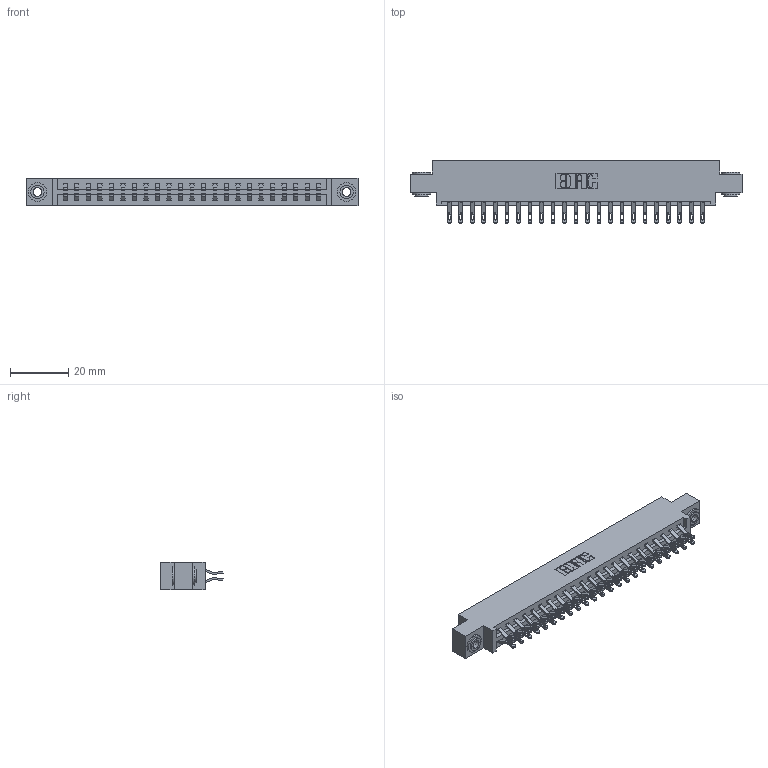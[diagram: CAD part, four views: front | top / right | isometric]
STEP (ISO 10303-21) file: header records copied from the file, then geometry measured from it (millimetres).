
FILE_DESCRIPTION (( 'STEP AP203' ), '1' );
FILE_NAME ('387-046-555-803.STEP', '2019-10-18T08:10:55', ( '' ), ( '' ), 'SwSTEP 2.0', 'SolidWorks 2016', '' );
FILE_SCHEMA (( 'CONFIG_CONTROL_DESIGN' ));
Length unit declared in the file: inch
Products named in the file (4): 337 Part_0.170 Offset - 0.156 Dia-TH; 345-250-002_345-250-002-102; 387-046-555-803; 345-292-001_555 Tail
Assembly tree (49 placements, depth 2):
  387-046-555-803
    337 Part_0.170 Offset - 0.156 Dia-TH
    345-292-001_555 Tail  x46
    345-250-002_345-250-002-102  x2
Bounding box: 114.15 x 21.47 x 9.4 mm (x, y, z)
Volume: 11812.2 mm3; surface area: 14004.2 mm2
Topology: 49 solids, 49 shells, 2916 faces, 9093 edges, 6058 vertices
Faces by surface type: plane 1740, cylinder 1168, cone 8
Entity records: 21398 total; most frequent: CARTESIAN_POINT 3631, ORIENTED_EDGE 3530, DIRECTION 3127, EDGE_CURVE 1765, VECTOR 1593, LINE 1593, VERTEX_POINT 1174, AXIS2_PLACEMENT_3D 767
